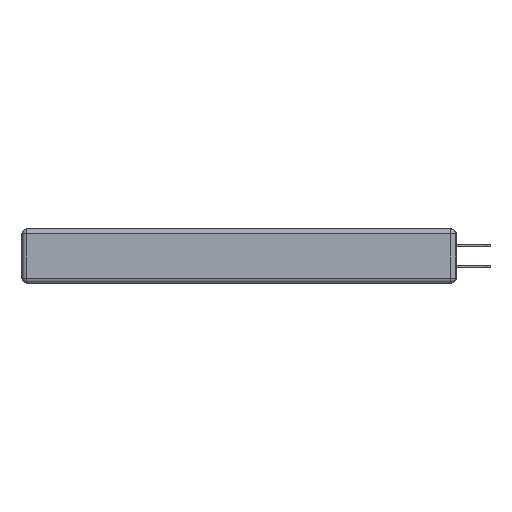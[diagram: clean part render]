
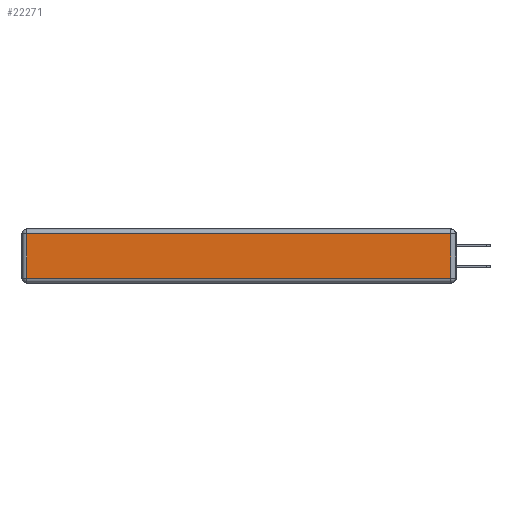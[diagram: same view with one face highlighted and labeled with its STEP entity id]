
A CAD part, left-side view. The second image highlights one B-rep face of the part: STEP entity #22271.
In plain terms, the highlighted planar face has unit normal (-1, 0, 0).
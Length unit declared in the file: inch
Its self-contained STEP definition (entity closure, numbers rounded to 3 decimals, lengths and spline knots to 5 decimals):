
#894 = CARTESIAN_POINT ( 'NONE',  ( 0., 0., -0.343 ) ) ;
#1039 = CARTESIAN_POINT ( 'NONE',  ( 0., 2.72, -0.03 ) ) ;
#1336 = VECTOR ( 'NONE', #8551, 39.37008 ) ;
#2127 = ORIENTED_EDGE ( 'NONE', *, *, #19049, .T. ) ;
#3064 = LINE ( 'NONE', #3819, #22121 ) ;
#3819 = CARTESIAN_POINT ( 'NONE',  ( 0., 2.72, -0.343 ) ) ;
#3878 = EDGE_CURVE ( 'NONE', #18587, #10508, #3064, .T. ) ;
#4177 = VERTEX_POINT ( 'NONE', #19149 ) ;
#6037 = CARTESIAN_POINT ( 'NONE',  ( 0., 2.75, -0.03 ) ) ;
#6222 = PLANE ( 'NONE',  #14524 ) ;
#6230 = VECTOR ( 'NONE', #16674, 39.37008 ) ;
#6498 = EDGE_LOOP ( 'NONE', ( #19716, #14068, #2127, #12110 ) ) ;
#6647 = EDGE_CURVE ( 'NONE', #4177, #9417, #16944, .T. ) ;
#7032 = EDGE_CURVE ( 'NONE', #10508, #4177, #14973, .T. ) ;
#8011 = DIRECTION ( 'NONE',  ( 0., 0., 1. ) ) ;
#8324 = CARTESIAN_POINT ( 'NONE',  ( 0., 0.03, -0.343 ) ) ;
#8551 = DIRECTION ( 'NONE',  ( 0., 0., 1. ) ) ;
#9168 = CARTESIAN_POINT ( 'NONE',  ( 0., 2.72, -0.313 ) ) ;
#9417 = VERTEX_POINT ( 'NONE', #16312 ) ;
#10010 = FACE_OUTER_BOUND ( 'NONE', #6498, .T. ) ;
#10508 = VERTEX_POINT ( 'NONE', #9168 ) ;
#10979 = LINE ( 'NONE', #6037, #6230 ) ;
#12110 = ORIENTED_EDGE ( 'NONE', *, *, #3878, .T. ) ;
#12533 = DIRECTION ( 'NONE',  ( 0., -1., 0. ) ) ;
#12609 = DIRECTION ( 'NONE',  ( 0., 0., -1. ) ) ;
#13426 = DIRECTION ( 'NONE',  ( -1., 0., 0. ) ) ;
#14068 = ORIENTED_EDGE ( 'NONE', *, *, #6647, .T. ) ;
#14205 = CARTESIAN_POINT ( 'NONE',  ( 0., 0., -0.313 ) ) ;
#14402 = VECTOR ( 'NONE', #12533, 39.37008 ) ;
#14524 = AXIS2_PLACEMENT_3D ( 'NONE', #894, #13426, #8011 ) ;
#14973 = LINE ( 'NONE', #14205, #14402 ) ;
#16312 = CARTESIAN_POINT ( 'NONE',  ( 0., 0.03, -0.03 ) ) ;
#16674 = DIRECTION ( 'NONE',  ( 0., 1., 0. ) ) ;
#16944 = LINE ( 'NONE', #8324, #1336 ) ;
#18587 = VERTEX_POINT ( 'NONE', #1039 ) ;
#19049 = EDGE_CURVE ( 'NONE', #9417, #18587, #10979, .T. ) ;
#19149 = CARTESIAN_POINT ( 'NONE',  ( 0., 0.03, -0.313 ) ) ;
#19716 = ORIENTED_EDGE ( 'NONE', *, *, #7032, .T. ) ;
#22121 = VECTOR ( 'NONE', #12609, 39.37008 ) ;
#22271 = ADVANCED_FACE ( 'NONE', ( #10010 ), #6222, .T. ) ;
